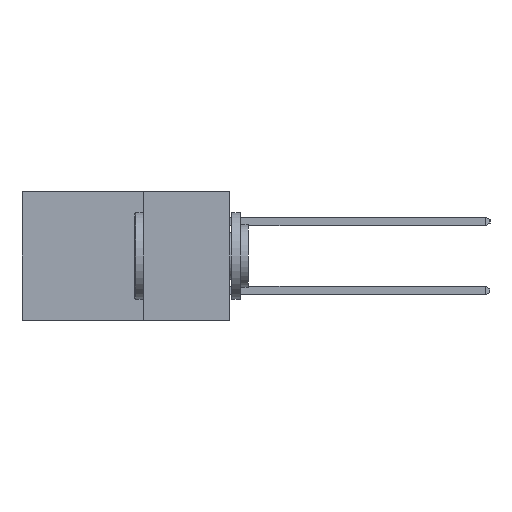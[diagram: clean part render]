
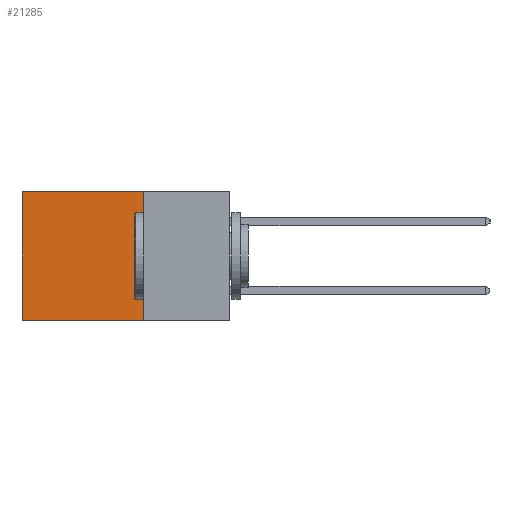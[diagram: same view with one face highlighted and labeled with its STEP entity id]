
A CAD part, left-side view. The second image highlights one B-rep face of the part: STEP entity #21285.
In plain terms, the highlighted planar face has unit normal (-1, 0, 0).
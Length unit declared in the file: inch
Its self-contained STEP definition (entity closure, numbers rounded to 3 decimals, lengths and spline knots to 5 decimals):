
#281 = CARTESIAN_POINT ( 'NONE',  ( 0.298, 0.25, 0. ) ) ;
#1668 = ORIENTED_EDGE ( 'NONE', *, *, #15080, .T. ) ;
#1857 = CARTESIAN_POINT ( 'NONE',  ( 0.298, 0.25, -0.37 ) ) ;
#1949 = FACE_OUTER_BOUND ( 'NONE', #28497, .T. ) ;
#2981 = VERTEX_POINT ( 'NONE', #17435 ) ;
#3532 = VERTEX_POINT ( 'NONE', #15084 ) ;
#3953 = LINE ( 'NONE', #27672, #22397 ) ;
#5009 = ORIENTED_EDGE ( 'NONE', *, *, #31087, .F. ) ;
#5608 = DIRECTION ( 'NONE',  ( 0., 0., -1. ) ) ;
#5788 = DIRECTION ( 'NONE',  ( 1., 0., 0. ) ) ;
#7492 = VERTEX_POINT ( 'NONE', #10976 ) ;
#9637 = CARTESIAN_POINT ( 'NONE',  ( 0.298, 0.6, 0. ) ) ;
#10976 = CARTESIAN_POINT ( 'NONE',  ( 0.298, 0.6, -0.37 ) ) ;
#13447 = ORIENTED_EDGE ( 'NONE', *, *, #18991, .F. ) ;
#15080 = EDGE_CURVE ( 'NONE', #3532, #26296, #24674, .T. ) ;
#15084 = CARTESIAN_POINT ( 'NONE',  ( 0.298, 0.25, 0. ) ) ;
#15347 = PLANE ( 'NONE',  #26262 ) ;
#15690 = DIRECTION ( 'NONE',  ( 0., 0., -1. ) ) ;
#15713 = VECTOR ( 'NONE', #5608, 39.37008 ) ;
#17435 = CARTESIAN_POINT ( 'NONE',  ( 0.298, 0.25, -0.37 ) ) ;
#18991 = EDGE_CURVE ( 'NONE', #3532, #2981, #3953, .T. ) ;
#20004 = CARTESIAN_POINT ( 'NONE',  ( 0.298, 0.6, 0. ) ) ;
#20198 = CARTESIAN_POINT ( 'NONE',  ( 0.298, 0.25, 0. ) ) ;
#21144 = DIRECTION ( 'NONE',  ( 0., 1., 0. ) ) ;
#21285 = ADVANCED_FACE ( 'NONE', ( #1949 ), #15347, .F. ) ;
#21361 = LINE ( 'NONE', #20004, #15713 ) ;
#21875 = DIRECTION ( 'NONE',  ( 0., 1., 0. ) ) ;
#22282 = ORIENTED_EDGE ( 'NONE', *, *, #27089, .T. ) ;
#22397 = VECTOR ( 'NONE', #15690, 39.37008 ) ;
#22555 = VECTOR ( 'NONE', #21144, 39.37008 ) ;
#22605 = DIRECTION ( 'NONE',  ( 0., 0., -1. ) ) ;
#24674 = LINE ( 'NONE', #281, #31027 ) ;
#26262 = AXIS2_PLACEMENT_3D ( 'NONE', #20198, #5788, #22605 ) ;
#26296 = VERTEX_POINT ( 'NONE', #9637 ) ;
#27089 = EDGE_CURVE ( 'NONE', #26296, #7492, #21361, .T. ) ;
#27672 = CARTESIAN_POINT ( 'NONE',  ( 0.298, 0.25, 0. ) ) ;
#28497 = EDGE_LOOP ( 'NONE', ( #22282, #5009, #13447, #1668 ) ) ;
#28925 = LINE ( 'NONE', #1857, #22555 ) ;
#31027 = VECTOR ( 'NONE', #21875, 39.37008 ) ;
#31087 = EDGE_CURVE ( 'NONE', #2981, #7492, #28925, .T. ) ;
